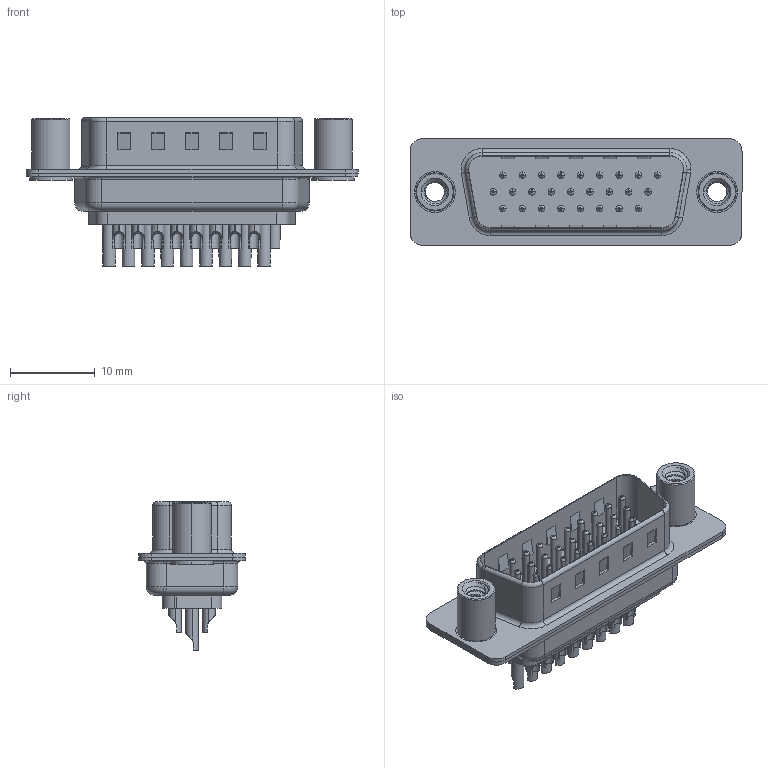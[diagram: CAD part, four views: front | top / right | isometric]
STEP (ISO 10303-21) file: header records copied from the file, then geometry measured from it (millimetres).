
FILE_DESCRIPTION (( 'STEP AP203' ), '1' );
FILE_NAME ('637-026-332-069.STEP', '2020-07-18T01:01:11', ( '' ), ( '' ), 'SwSTEP 2.0', 'SolidWorks 2020', '' );
FILE_SCHEMA (( 'CONFIG_CONTROL_DESIGN' ));
Length unit declared in the file: millimetre
Products named in the file (8): 637 Shell Front_26 Contacts; 637-026-332-069; 637 Contact Row 3_32; 637 Contact Row 2_32; 637 4-40 Threaded Standoff; 637 Shell Rear_26 Contacts; 637 Contact Row 1_32; 637 Housing_26 Contacts
Assembly tree (31 placements, depth 2):
  637-026-332-069
    637 Housing_26 Contacts
    637 Shell Front_26 Contacts
    637 Shell Rear_26 Contacts
    637 Contact Row 1_32  x9
    637 Contact Row 2_32  x9
    637 Contact Row 3_32  x8
    637 4-40 Threaded Standoff  x2
Bounding box: 39.2 x 12.6 x 17.55 mm (x, y, z)
Volume: 1917.6 mm3; surface area: 7120.4 mm2
Topology: 31 solids, 31 shells, 2038 faces, 5213 edges, 3302 vertices
Faces by surface type: cylinder 915, torus 596, plane 505, cone 16, bspline 6
Entity records: 24364 total; most frequent: CARTESIAN_POINT 5511, DIRECTION 3934, ORIENTED_EDGE 3456, EDGE_CURVE 1728, AXIS2_PLACEMENT_3D 1582, VERTEX_POINT 1104, CIRCLE 851, EDGE_LOOP 848
